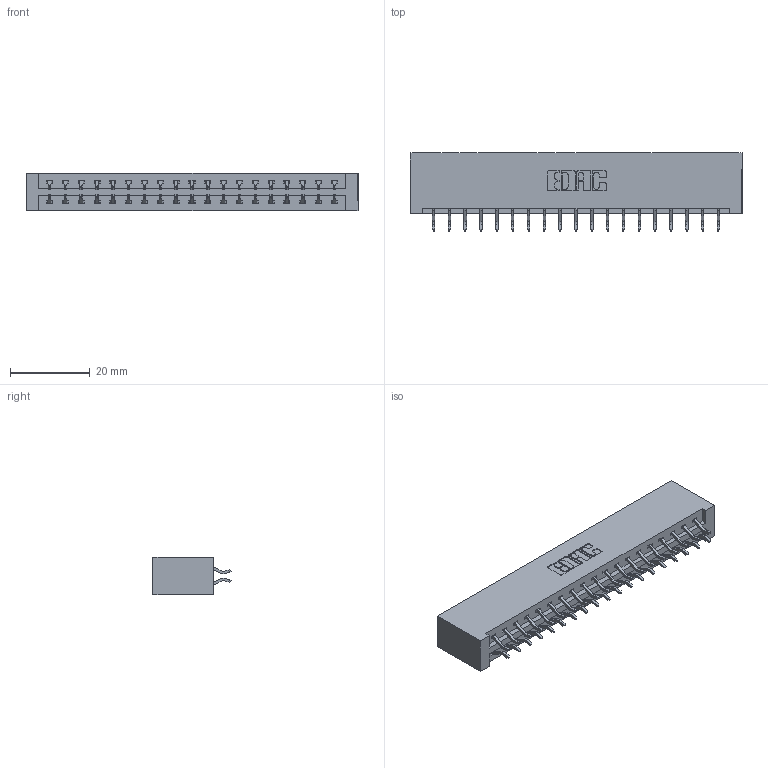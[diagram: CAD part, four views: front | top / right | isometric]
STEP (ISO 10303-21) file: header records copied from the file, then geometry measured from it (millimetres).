
FILE_DESCRIPTION (( 'STEP AP203' ), '1' );
FILE_NAME ('337-038-556-201.STEP', '2019-10-09T11:02:54', ( '' ), ( '' ), 'SwSTEP 2.0', 'SolidWorks 2016', '' );
FILE_SCHEMA (( 'CONFIG_CONTROL_DESIGN' ));
Length unit declared in the file: inch
Products named in the file (3): 337-038-556-201; 345-292-001_556 Tail; 337 Part_No Mounting Lugs
Assembly tree (39 placements, depth 2):
  337-038-556-201
    337 Part_No Mounting Lugs
    345-292-001_556 Tail  x38
Bounding box: 83.16 x 19.57 x 9.4 mm (x, y, z)
Volume: 9217.1 mm3; surface area: 10212.5 mm2
Topology: 39 solids, 39 shells, 2386 faces, 7089 edges, 4674 vertices
Faces by surface type: plane 1662, cylinder 724
Entity records: 17649 total; most frequent: CARTESIAN_POINT 3006, ORIENTED_EDGE 2930, DIRECTION 2581, EDGE_CURVE 1465, VECTOR 1337, LINE 1337, VERTEX_POINT 974, AXIS2_PLACEMENT_3D 622
